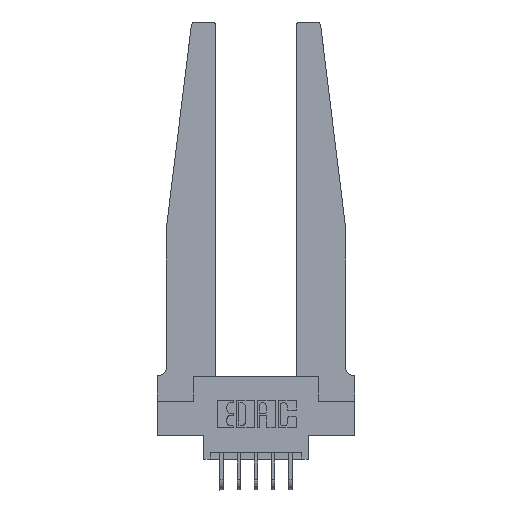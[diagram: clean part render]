
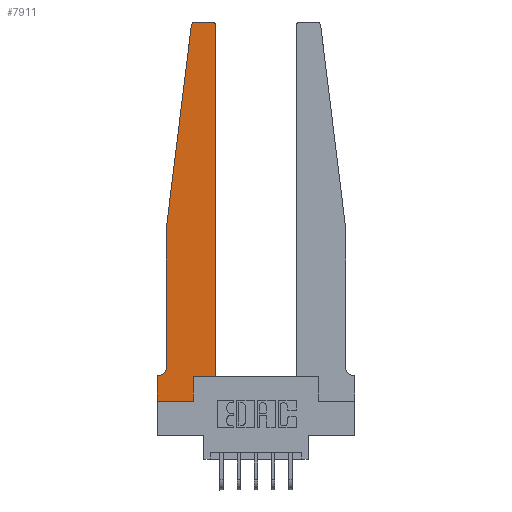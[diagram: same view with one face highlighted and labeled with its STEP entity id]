
A CAD part, top view. The second image highlights one B-rep face of the part: STEP entity #7911.
In plain terms, the highlighted planar face has unit normal (0, 0, 1).
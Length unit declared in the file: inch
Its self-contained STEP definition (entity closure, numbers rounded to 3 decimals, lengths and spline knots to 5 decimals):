
#15 = AXIS2_PLACEMENT_3D ( 'NONE', #410, #14647, #4153 ) ;
#191 = DIRECTION ( 'NONE',  ( 0., 1., 0. ) ) ;
#271 = DIRECTION ( 'NONE',  ( 0., 0., -1. ) ) ;
#282 = ORIENTED_EDGE ( 'NONE', *, *, #5657, .T. ) ;
#378 = CARTESIAN_POINT ( 'NONE',  ( 0.395, 2.75, 0.37 ) ) ;
#410 = CARTESIAN_POINT ( 'NONE',  ( 0.27653, 2.72, 0.37 ) ) ;
#461 = AXIS2_PLACEMENT_3D ( 'NONE', #5550, #5833, #12536 ) ;
#472 = VECTOR ( 'NONE', #10089, 39.37008 ) ;
#677 = CARTESIAN_POINT ( 'NONE',  ( 0.395, 2.72, 0.37 ) ) ;
#1174 = CARTESIAN_POINT ( 'NONE',  ( 0.25, 2.75, 0.37 ) ) ;
#1212 = VECTOR ( 'NONE', #6471, 39.37008 ) ;
#1264 = VERTEX_POINT ( 'NONE', #4259 ) ;
#1306 = ORIENTED_EDGE ( 'NONE', *, *, #9110, .T. ) ;
#1418 = LINE ( 'NONE', #1174, #7218 ) ;
#1458 = CARTESIAN_POINT ( 'NONE',  ( 0., 0., 0.37 ) ) ;
#1661 = DIRECTION ( 'NONE',  ( 1., 0., 0. ) ) ;
#1707 = CARTESIAN_POINT ( 'NONE',  ( 0.2605, 0., 0.37 ) ) ;
#2321 = EDGE_CURVE ( 'NONE', #3870, #7111, #7063, .T. ) ;
#2403 = EDGE_CURVE ( 'NONE', #1264, #3870, #13989, .T. ) ;
#2566 = CARTESIAN_POINT ( 'NONE',  ( 0., 0.1875, 0.37 ) ) ;
#2753 = CARTESIAN_POINT ( 'NONE',  ( 0.015, 0.1875, 0.37 ) ) ;
#2900 = LINE ( 'NONE', #8376, #1212 ) ;
#3053 = VECTOR ( 'NONE', #10604, 39.37008 ) ;
#3171 = CARTESIAN_POINT ( 'NONE',  ( 0.425, 0.18, 0.37 ) ) ;
#3242 = CIRCLE ( 'NONE', #15, 0.03 ) ;
#3339 = CARTESIAN_POINT ( 'NONE',  ( 0.425, 0.18, 0.37 ) ) ;
#3579 = ORIENTED_EDGE ( 'NONE', *, *, #2403, .T. ) ;
#3581 = CARTESIAN_POINT ( 'NONE',  ( 0.065, 1.25, 0.37 ) ) ;
#3620 = DIRECTION ( 'NONE',  ( 0., -1., 0. ) ) ;
#3703 = VERTEX_POINT ( 'NONE', #10124 ) ;
#3725 = LINE ( 'NONE', #3581, #12154 ) ;
#3870 = VERTEX_POINT ( 'NONE', #2753 ) ;
#4153 = DIRECTION ( 'NONE',  ( 1., 0., 0. ) ) ;
#4259 = CARTESIAN_POINT ( 'NONE',  ( 0.065, 0.2375, 0.37 ) ) ;
#4313 = FACE_OUTER_BOUND ( 'NONE', #15142, .T. ) ;
#4353 = LINE ( 'NONE', #3171, #472 ) ;
#4728 = VECTOR ( 'NONE', #191, 39.37008 ) ;
#4904 = VERTEX_POINT ( 'NONE', #7241 ) ;
#5233 = AXIS2_PLACEMENT_3D ( 'NONE', #677, #7611, #8845 ) ;
#5346 = CARTESIAN_POINT ( 'NONE',  ( 0.27653, 2.75, 0.37 ) ) ;
#5505 = ORIENTED_EDGE ( 'NONE', *, *, #9862, .T. ) ;
#5548 = ORIENTED_EDGE ( 'NONE', *, *, #2321, .T. ) ;
#5550 = CARTESIAN_POINT ( 'NONE',  ( 0., 0.1875, 0.37 ) ) ;
#5657 = EDGE_CURVE ( 'NONE', #7549, #6854, #8198, .T. ) ;
#5833 = DIRECTION ( 'NONE',  ( 0., 0., 1. ) ) ;
#5877 = CARTESIAN_POINT ( 'NONE',  ( 0.2605, 0.18, 0.37 ) ) ;
#6105 = CARTESIAN_POINT ( 'NONE',  ( 0.425, 2.72, 0.37 ) ) ;
#6471 = DIRECTION ( 'NONE',  ( -0.122, -0.992, 0. ) ) ;
#6538 = EDGE_CURVE ( 'NONE', #11116, #6957, #12582, .T. ) ;
#6854 = VERTEX_POINT ( 'NONE', #378 ) ;
#6957 = VERTEX_POINT ( 'NONE', #3339 ) ;
#7063 = LINE ( 'NONE', #11842, #3053 ) ;
#7111 = VERTEX_POINT ( 'NONE', #2566 ) ;
#7214 = DIRECTION ( 'NONE',  ( -1., 0., 0. ) ) ;
#7218 = VECTOR ( 'NONE', #9617, 39.37008 ) ;
#7241 = CARTESIAN_POINT ( 'NONE',  ( 0.24675, 2.72367, 0.37 ) ) ;
#7450 = ORIENTED_EDGE ( 'NONE', *, *, #9851, .T. ) ;
#7549 = VERTEX_POINT ( 'NONE', #6105 ) ;
#7611 = DIRECTION ( 'NONE',  ( 0., 0., 1. ) ) ;
#7789 = CARTESIAN_POINT ( 'NONE',  ( 0.065, 1.25, 0.37 ) ) ;
#7811 = PLANE ( 'NONE',  #461 ) ;
#7911 = ADVANCED_FACE ( 'NONE', ( #4313 ), #7811, .T. ) ;
#8198 = CIRCLE ( 'NONE', #5233, 0.03 ) ;
#8232 = EDGE_CURVE ( 'NONE', #6957, #7549, #4353, .T. ) ;
#8376 = CARTESIAN_POINT ( 'NONE',  ( 0.065, 1.25, 0.37 ) ) ;
#8468 = DIRECTION ( 'NONE',  ( 0., -1., 0. ) ) ;
#8683 = VECTOR ( 'NONE', #3620, 39.37008 ) ;
#8830 = EDGE_CURVE ( 'NONE', #7111, #3703, #10913, .T. ) ;
#8845 = DIRECTION ( 'NONE',  ( 1., 0., 0. ) ) ;
#8850 = LINE ( 'NONE', #13586, #11949 ) ;
#8867 = EDGE_CURVE ( 'NONE', #10853, #11116, #14201, .T. ) ;
#9006 = ORIENTED_EDGE ( 'NONE', *, *, #13280, .T. ) ;
#9110 = EDGE_CURVE ( 'NONE', #14562, #4904, #3242, .T. ) ;
#9617 = DIRECTION ( 'NONE',  ( -1., 0., 0. ) ) ;
#9821 = CARTESIAN_POINT ( 'NONE',  ( 0.015, 0.2375, 0.37 ) ) ;
#9851 = EDGE_CURVE ( 'NONE', #6854, #14562, #1418, .T. ) ;
#9862 = EDGE_CURVE ( 'NONE', #12309, #1264, #3725, .T. ) ;
#9950 = CARTESIAN_POINT ( 'NONE',  ( 0.425, 0.18, 0.37 ) ) ;
#10089 = DIRECTION ( 'NONE',  ( 0., 1., 0. ) ) ;
#10124 = CARTESIAN_POINT ( 'NONE',  ( 0., 0., 0.37 ) ) ;
#10177 = ORIENTED_EDGE ( 'NONE', *, *, #6538, .T. ) ;
#10414 = ORIENTED_EDGE ( 'NONE', *, *, #8867, .T. ) ;
#10464 = ORIENTED_EDGE ( 'NONE', *, *, #8830, .T. ) ;
#10604 = DIRECTION ( 'NONE',  ( -1., 0., 0. ) ) ;
#10853 = VERTEX_POINT ( 'NONE', #1707 ) ;
#10913 = LINE ( 'NONE', #1458, #8683 ) ;
#11116 = VERTEX_POINT ( 'NONE', #5877 ) ;
#11412 = DIRECTION ( 'NONE',  ( 1., 0., 0. ) ) ;
#11842 = CARTESIAN_POINT ( 'NONE',  ( 0.065, 0.1875, 0.37 ) ) ;
#11949 = VECTOR ( 'NONE', #11412, 39.37008 ) ;
#11994 = AXIS2_PLACEMENT_3D ( 'NONE', #9821, #271, #7214 ) ;
#12008 = CARTESIAN_POINT ( 'NONE',  ( 0.2605, 0.18, 0.37 ) ) ;
#12154 = VECTOR ( 'NONE', #8468, 39.37008 ) ;
#12309 = VERTEX_POINT ( 'NONE', #7789 ) ;
#12536 = DIRECTION ( 'NONE',  ( 1., 0., 0. ) ) ;
#12582 = LINE ( 'NONE', #9950, #12925 ) ;
#12905 = ORIENTED_EDGE ( 'NONE', *, *, #8232, .T. ) ;
#12925 = VECTOR ( 'NONE', #1661, 39.37008 ) ;
#13280 = EDGE_CURVE ( 'NONE', #4904, #12309, #2900, .T. ) ;
#13321 = ORIENTED_EDGE ( 'NONE', *, *, #14141, .T. ) ;
#13586 = CARTESIAN_POINT ( 'NONE',  ( 0., 0., 0.37 ) ) ;
#13989 = CIRCLE ( 'NONE', #11994, 0.05 ) ;
#14141 = EDGE_CURVE ( 'NONE', #3703, #10853, #8850, .T. ) ;
#14201 = LINE ( 'NONE', #12008, #4728 ) ;
#14562 = VERTEX_POINT ( 'NONE', #5346 ) ;
#14647 = DIRECTION ( 'NONE',  ( 0., 0., 1. ) ) ;
#15142 = EDGE_LOOP ( 'NONE', ( #7450, #1306, #9006, #5505, #3579, #5548, #10464, #13321, #10414, #10177, #12905, #282 ) ) ;
